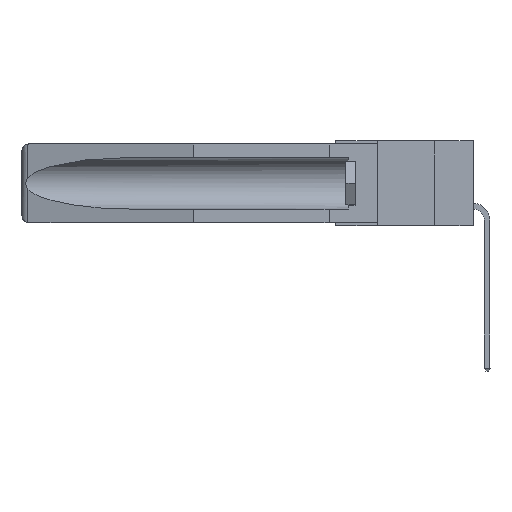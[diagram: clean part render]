
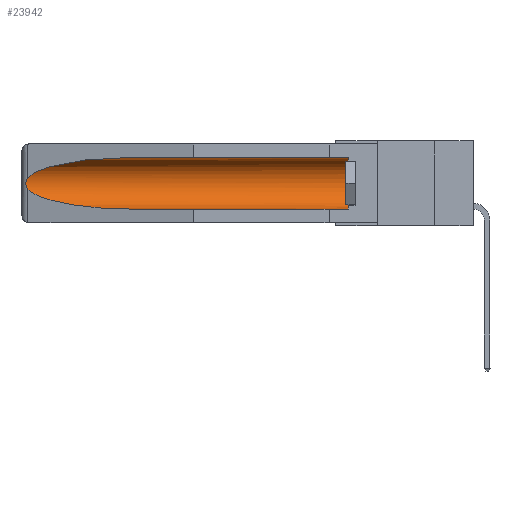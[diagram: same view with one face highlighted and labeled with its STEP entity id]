
A CAD part, left-side view. The second image highlights one B-rep face of the part: STEP entity #23942.
In plain terms, the highlighted cylindrical face has radius 2.857 mm (diameter 5.715 mm), a partial arc.
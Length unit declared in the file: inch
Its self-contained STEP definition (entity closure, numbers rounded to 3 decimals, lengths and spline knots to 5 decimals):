
#886 = CARTESIAN_POINT ( 'NONE',  ( 0.2675, 1.53308, -0.17534 ) ) ;
#1488 = VECTOR ( 'NONE', #10833, 39.37008 ) ;
#2279 = DIRECTION ( 'NONE',  ( 0., 0., 1. ) ) ;
#2750 = CARTESIAN_POINT ( 'NONE',  ( 0.26537, 1.52718, -0.14972 ) ) ;
#3573 = ORIENTED_EDGE ( 'NONE', *, *, #15243, .T. ) ;
#3721 = CARTESIAN_POINT ( 'NONE',  ( 0.155, 1.07973, -0.284 ) ) ;
#3844 = B_SPLINE_CURVE_WITH_KNOTS ( 'NONE', 3,
 ( #20839, #7671, #15626, #8300, #10155, #886, #8367, #13829, #15710, #17621 ),
 .UNSPECIFIED., .F., .F.,
 ( 4, 2, 2, 2, 4 ),
 ( 0., 0.00029, 0.00058, 0.00087, 0.00117 ),
 .UNSPECIFIED. ) ;
#4066 = DIRECTION ( 'NONE',  ( 0., 0., 1. ) ) ;
#4171 = VERTEX_POINT ( 'NONE', #22371 ) ;
#5601 = VERTEX_POINT ( 'NONE', #8792 ) ;
#5655 = DIRECTION ( 'NONE',  ( 0., 1., 0. ) ) ;
#6879 = ORIENTED_EDGE ( 'NONE', *, *, #18825, .T. ) ;
#7319 = CARTESIAN_POINT ( 'NONE',  ( 0.26537, 1.52718, -0.19328 ) ) ;
#7671 = CARTESIAN_POINT ( 'NONE',  ( 0.26597, 1.52961, -0.15275 ) ) ;
#8027 = EDGE_CURVE ( 'NONE', #16307, #5601, #21250, .T. ) ;
#8300 = CARTESIAN_POINT ( 'NONE',  ( 0.2673, 1.5327, -0.16383 ) ) ;
#8367 = CARTESIAN_POINT ( 'NONE',  ( 0.2673, 1.53269, -0.17917 ) ) ;
#8792 = CARTESIAN_POINT ( 'NONE',  ( 0.155, 1.07973, -0.284 ) ) ;
#8798 = ORIENTED_EDGE ( 'NONE', *, *, #22174, .T. ) ;
#10155 = CARTESIAN_POINT ( 'NONE',  ( 0.2675, 1.53308, -0.16763 ) ) ;
#10435 = VECTOR ( 'NONE', #21893, 39.37008 ) ;
#10729 = CARTESIAN_POINT ( 'NONE',  ( 0.155, -0.30754, -0.059 ) ) ;
#10833 = DIRECTION ( 'NONE',  ( 0., 1., 0. ) ) ;
#11002 = CARTESIAN_POINT ( 'NONE',  ( 0.155, -0.30754, -0.284 ) ) ;
#11149 = VERTEX_POINT ( 'NONE', #11531 ) ;
#11531 = CARTESIAN_POINT ( 'NONE',  ( 0.26537, 1.52718, -0.19328 ) ) ;
#11860 = CARTESIAN_POINT ( 'NONE',  ( 0.155, 1.07973, -0.059 ) ) ;
#12213 = ORIENTED_EDGE ( 'NONE', *, *, #22895, .T. ) ;
#12419 = EDGE_CURVE ( 'NONE', #11149, #5601, #13899, .T. ) ;
#13202 = CARTESIAN_POINT ( 'NONE',  ( 0.26537, 1.52718, -0.14972 ) ) ;
#13781 = ORIENTED_EDGE ( 'NONE', *, *, #8027, .F. ) ;
#13829 = CARTESIAN_POINT ( 'NONE',  ( 0.26655, 1.53094, -0.18657 ) ) ;
#13899 =( BOUNDED_CURVE ( )  B_SPLINE_CURVE ( 3, ( #7319, #23860, #16703, #3721 ),
 .UNSPECIFIED., .F., .F. ) 
 B_SPLINE_CURVE_WITH_KNOTS ( ( 4, 4 ),
 ( 0.1948, 1.5708 ),
 .UNSPECIFIED. ) 
 CURVE ( )  GEOMETRIC_REPRESENTATION_ITEM ( )  RATIONAL_B_SPLINE_CURVE ( ( 1., 0.848, 0.848, 1. ) ) 
 REPRESENTATION_ITEM ( '' )  );
#14625 = VERTEX_POINT ( 'NONE', #13202 ) ;
#14873 = CARTESIAN_POINT ( 'NONE',  ( 0.155, -0.30754, -0.1715 ) ) ;
#14969 = EDGE_LOOP ( 'NONE', ( #12213, #3573, #21959, #13781, #8798, #6879 ) ) ;
#15243 = EDGE_CURVE ( 'NONE', #14625, #11149, #3844, .T. ) ;
#15626 = CARTESIAN_POINT ( 'NONE',  ( 0.26654, 1.53092, -0.15636 ) ) ;
#15710 = CARTESIAN_POINT ( 'NONE',  ( 0.26597, 1.5296, -0.19026 ) ) ;
#16307 = VERTEX_POINT ( 'NONE', #19877 ) ;
#16703 = CARTESIAN_POINT ( 'NONE',  ( 0.21114, 1.30732, -0.284 ) ) ;
#17304 = CARTESIAN_POINT ( 'NONE',  ( 0.155, 0.126, -0.1715 ) ) ;
#17621 = CARTESIAN_POINT ( 'NONE',  ( 0.26537, 1.52718, -0.19328 ) ) ;
#17914 = CYLINDRICAL_SURFACE ( 'NONE', #20988, 0.1125 ) ;
#18307 =( BOUNDED_CURVE ( )  B_SPLINE_CURVE ( 3, ( #19463, #23416, #21336, #2750 ),
 .UNSPECIFIED., .F., .F. ) 
 B_SPLINE_CURVE_WITH_KNOTS ( ( 4, 4 ),
 ( 4.71239, 6.08839 ),
 .UNSPECIFIED. ) 
 CURVE ( )  GEOMETRIC_REPRESENTATION_ITEM ( )  RATIONAL_B_SPLINE_CURVE ( ( 1., 0.848, 0.848, 1. ) ) 
 REPRESENTATION_ITEM ( '' )  );
#18825 = EDGE_CURVE ( 'NONE', #4171, #20937, #20366, .T. ) ;
#19249 = AXIS2_PLACEMENT_3D ( 'NONE', #17304, #20831, #4066 ) ;
#19463 = CARTESIAN_POINT ( 'NONE',  ( 0.155, 1.07973, -0.059 ) ) ;
#19877 = CARTESIAN_POINT ( 'NONE',  ( 0.155, 0.126, -0.284 ) ) ;
#20366 = LINE ( 'NONE', #10729, #10435 ) ;
#20831 = DIRECTION ( 'NONE',  ( 0., -1., 0. ) ) ;
#20839 = CARTESIAN_POINT ( 'NONE',  ( 0.26537, 1.52718, -0.14972 ) ) ;
#20937 = VERTEX_POINT ( 'NONE', #11860 ) ;
#20988 = AXIS2_PLACEMENT_3D ( 'NONE', #14873, #5655, #2279 ) ;
#21250 = LINE ( 'NONE', #11002, #1488 ) ;
#21336 = CARTESIAN_POINT ( 'NONE',  ( 0.25451, 1.48313, -0.09465 ) ) ;
#21569 = CIRCLE ( 'NONE', #19249, 0.1125 ) ;
#21893 = DIRECTION ( 'NONE',  ( 0., 1., 0. ) ) ;
#21959 = ORIENTED_EDGE ( 'NONE', *, *, #12419, .T. ) ;
#22174 = EDGE_CURVE ( 'NONE', #16307, #4171, #21569, .T. ) ;
#22371 = CARTESIAN_POINT ( 'NONE',  ( 0.155, 0.126, -0.059 ) ) ;
#22895 = EDGE_CURVE ( 'NONE', #20937, #14625, #18307, .T. ) ;
#23413 = FACE_OUTER_BOUND ( 'NONE', #14969, .T. ) ;
#23416 = CARTESIAN_POINT ( 'NONE',  ( 0.21114, 1.30732, -0.059 ) ) ;
#23860 = CARTESIAN_POINT ( 'NONE',  ( 0.25451, 1.48313, -0.24835 ) ) ;
#23942 = ADVANCED_FACE ( 'NONE', ( #23413 ), #17914, .F. ) ;
